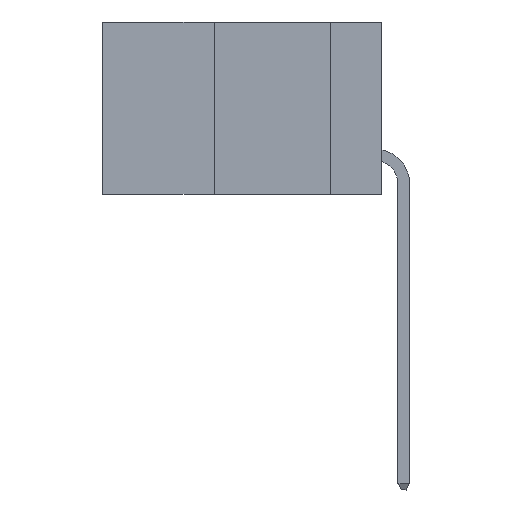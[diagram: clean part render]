
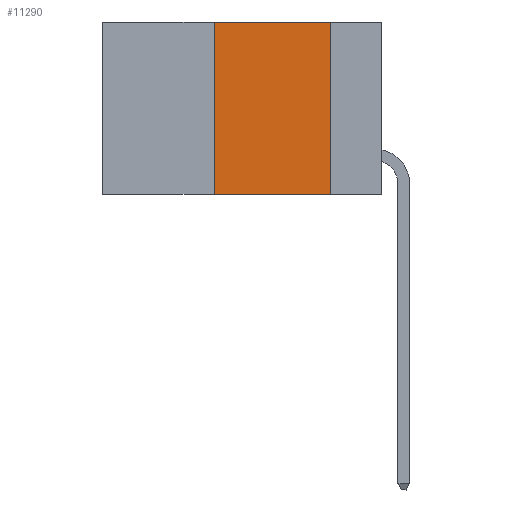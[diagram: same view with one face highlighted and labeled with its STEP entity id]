
A CAD part, left-side view. The second image highlights one B-rep face of the part: STEP entity #11290.
In plain terms, the highlighted planar face has unit normal (-1, 0, 0).
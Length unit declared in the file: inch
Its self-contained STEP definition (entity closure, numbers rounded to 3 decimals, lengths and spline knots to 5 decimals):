
#74 = VERTEX_POINT ( 'NONE', #10593 ) ;
#283 = CARTESIAN_POINT ( 'NONE',  ( 0., 0.36, 0. ) ) ;
#326 = VERTEX_POINT ( 'NONE', #7252 ) ;
#1590 = LINE ( 'NONE', #4552, #3419 ) ;
#2088 = VECTOR ( 'NONE', #9081, 39.37008 ) ;
#2199 = VERTEX_POINT ( 'NONE', #12965 ) ;
#2266 = LINE ( 'NONE', #283, #9122 ) ;
#2413 = PLANE ( 'NONE',  #6038 ) ;
#2624 = ORIENTED_EDGE ( 'NONE', *, *, #12778, .F. ) ;
#2627 = ORIENTED_EDGE ( 'NONE', *, *, #2710, .F. ) ;
#2634 = DIRECTION ( 'NONE',  ( 0., -1., 0. ) ) ;
#2710 = EDGE_CURVE ( 'NONE', #2199, #74, #4359, .T. ) ;
#3041 = EDGE_CURVE ( 'NONE', #11321, #74, #6024, .T. ) ;
#3419 = VECTOR ( 'NONE', #2634, 39.37008 ) ;
#3522 = DIRECTION ( 'NONE',  ( 0., 0., -1. ) ) ;
#4359 = LINE ( 'NONE', #6335, #7042 ) ;
#4552 = CARTESIAN_POINT ( 'NONE',  ( 0., 0.6, 0. ) ) ;
#5131 = EDGE_CURVE ( 'NONE', #326, #2199, #1590, .T. ) ;
#5504 = FACE_OUTER_BOUND ( 'NONE', #10118, .T. ) ;
#6024 = LINE ( 'NONE', #11283, #2088 ) ;
#6038 = AXIS2_PLACEMENT_3D ( 'NONE', #12612, #11612, #3522 ) ;
#6335 = CARTESIAN_POINT ( 'NONE',  ( 0., 0.11, 0. ) ) ;
#6887 = ORIENTED_EDGE ( 'NONE', *, *, #5131, .F. ) ;
#7042 = VECTOR ( 'NONE', #12588, 39.37008 ) ;
#7252 = CARTESIAN_POINT ( 'NONE',  ( 0., 0.36, 0. ) ) ;
#9081 = DIRECTION ( 'NONE',  ( 0., -1., 0. ) ) ;
#9122 = VECTOR ( 'NONE', #12074, 39.37008 ) ;
#10118 = EDGE_LOOP ( 'NONE', ( #2627, #6887, #2624, #10625 ) ) ;
#10593 = CARTESIAN_POINT ( 'NONE',  ( 0., 0.11, -0.37 ) ) ;
#10625 = ORIENTED_EDGE ( 'NONE', *, *, #3041, .T. ) ;
#11283 = CARTESIAN_POINT ( 'NONE',  ( 0., 0.6, -0.37 ) ) ;
#11290 = ADVANCED_FACE ( 'NONE', ( #5504 ), #2413, .F. ) ;
#11321 = VERTEX_POINT ( 'NONE', #13004 ) ;
#11612 = DIRECTION ( 'NONE',  ( 1., 0., 0. ) ) ;
#12074 = DIRECTION ( 'NONE',  ( 0., 0., 1. ) ) ;
#12588 = DIRECTION ( 'NONE',  ( 0., 0., -1. ) ) ;
#12612 = CARTESIAN_POINT ( 'NONE',  ( 0., 0.6, 0. ) ) ;
#12778 = EDGE_CURVE ( 'NONE', #11321, #326, #2266, .T. ) ;
#12965 = CARTESIAN_POINT ( 'NONE',  ( 0., 0.11, 0. ) ) ;
#13004 = CARTESIAN_POINT ( 'NONE',  ( 0., 0.36, -0.37 ) ) ;
